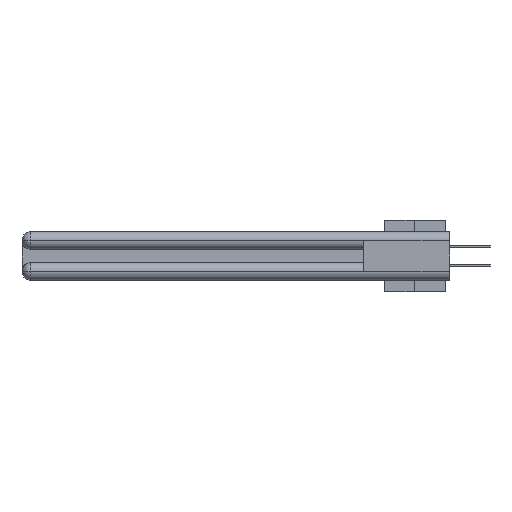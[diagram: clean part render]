
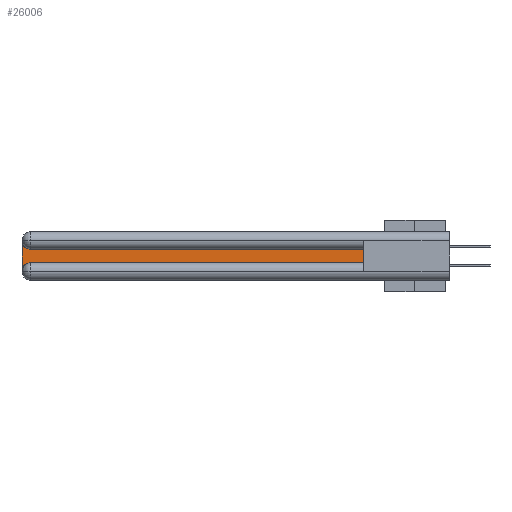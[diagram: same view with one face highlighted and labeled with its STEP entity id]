
A CAD part, left-side view. The second image highlights one B-rep face of the part: STEP entity #26006.
In plain terms, the highlighted planar face has unit normal (-1, 0, 0).
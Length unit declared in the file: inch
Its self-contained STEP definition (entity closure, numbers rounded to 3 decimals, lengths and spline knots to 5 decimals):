
#710 = PLANE ( 'NONE',  #14852 ) ;
#845 = DIRECTION ( 'NONE',  ( 1., 0., 0. ) ) ;
#1013 = EDGE_CURVE ( 'NONE', #38386, #38978, #7059, .T. ) ;
#2311 = DIRECTION ( 'NONE',  ( 1., 0., 0. ) ) ;
#3162 = ORIENTED_EDGE ( 'NONE', *, *, #1013, .T. ) ;
#3433 = VECTOR ( 'NONE', #27689, 39.37008 ) ;
#3435 = AXIS2_PLACEMENT_3D ( 'NONE', #39611, #2311, #8505 ) ;
#5744 = ORIENTED_EDGE ( 'NONE', *, *, #23359, .T. ) ;
#7059 = CIRCLE ( 'NONE', #3435, 0.06 ) ;
#7142 = CARTESIAN_POINT ( 'NONE',  ( 0.075, 3., -0.0625 ) ) ;
#8338 = DIRECTION ( 'NONE',  ( 0., 0., -1. ) ) ;
#8505 = DIRECTION ( 'NONE',  ( 0., 0., -1. ) ) ;
#8598 = CARTESIAN_POINT ( 'NONE',  ( 0.075, 0.6, -0.2175 ) ) ;
#9705 = VERTEX_POINT ( 'NONE', #8598 ) ;
#10027 = CARTESIAN_POINT ( 'NONE',  ( 0.075, 3., -0.1225 ) ) ;
#11762 = VERTEX_POINT ( 'NONE', #15130 ) ;
#12354 = EDGE_CURVE ( 'NONE', #9705, #26918, #33529, .T. ) ;
#12891 = DIRECTION ( 'NONE',  ( 0., -1., 0. ) ) ;
#14852 = AXIS2_PLACEMENT_3D ( 'NONE', #10027, #845, #31821 ) ;
#15130 = CARTESIAN_POINT ( 'NONE',  ( 0.075, 2.94, -0.2175 ) ) ;
#15148 = ORIENTED_EDGE ( 'NONE', *, *, #16966, .T. ) ;
#15164 = EDGE_CURVE ( 'NONE', #33441, #11762, #19171, .T. ) ;
#16138 = EDGE_LOOP ( 'NONE', ( #22279, #3162, #15148, #19310, #5744, #24178 ) ) ;
#16966 = EDGE_CURVE ( 'NONE', #38978, #33441, #19098, .T. ) ;
#17903 = AXIS2_PLACEMENT_3D ( 'NONE', #29203, #27306, #8338 ) ;
#19098 = LINE ( 'NONE', #36975, #3433 ) ;
#19171 = CIRCLE ( 'NONE', #17903, 0.06 ) ;
#19310 = ORIENTED_EDGE ( 'NONE', *, *, #15164, .T. ) ;
#20104 = CARTESIAN_POINT ( 'NONE',  ( 0.075, 3., -0.2775 ) ) ;
#20936 = LINE ( 'NONE', #26439, #37060 ) ;
#22279 = ORIENTED_EDGE ( 'NONE', *, *, #35531, .T. ) ;
#23154 = CARTESIAN_POINT ( 'NONE',  ( 0.075, 2.94, -0.1225 ) ) ;
#23359 = EDGE_CURVE ( 'NONE', #11762, #9705, #28509, .T. ) ;
#24178 = ORIENTED_EDGE ( 'NONE', *, *, #12354, .T. ) ;
#24619 = VECTOR ( 'NONE', #12891, 39.37008 ) ;
#25233 = CARTESIAN_POINT ( 'NONE',  ( 0.075, 0.6, -0.1225 ) ) ;
#26006 = ADVANCED_FACE ( 'NONE', ( #36746 ), #710, .F. ) ;
#26439 = CARTESIAN_POINT ( 'NONE',  ( 0.075, 0.6, -0.1225 ) ) ;
#26918 = VERTEX_POINT ( 'NONE', #25233 ) ;
#27306 = DIRECTION ( 'NONE',  ( 1., 0., 0. ) ) ;
#27516 = CARTESIAN_POINT ( 'NONE',  ( 0.075, 0.6, -0.2175 ) ) ;
#27689 = DIRECTION ( 'NONE',  ( 0., 0., -1. ) ) ;
#28509 = LINE ( 'NONE', #38287, #24619 ) ;
#29203 = CARTESIAN_POINT ( 'NONE',  ( 0.075, 2.94, -0.2775 ) ) ;
#30622 = DIRECTION ( 'NONE',  ( 0., 0., 1. ) ) ;
#31821 = DIRECTION ( 'NONE',  ( 0., 0., -1. ) ) ;
#33441 = VERTEX_POINT ( 'NONE', #20104 ) ;
#33529 = LINE ( 'NONE', #27516, #34500 ) ;
#34500 = VECTOR ( 'NONE', #30622, 39.37008 ) ;
#35531 = EDGE_CURVE ( 'NONE', #26918, #38386, #20936, .T. ) ;
#36746 = FACE_OUTER_BOUND ( 'NONE', #16138, .T. ) ;
#36975 = CARTESIAN_POINT ( 'NONE',  ( 0.075, 3., -0.2175 ) ) ;
#37060 = VECTOR ( 'NONE', #38725, 39.37008 ) ;
#38287 = CARTESIAN_POINT ( 'NONE',  ( 0.075, 0.6, -0.2175 ) ) ;
#38386 = VERTEX_POINT ( 'NONE', #23154 ) ;
#38725 = DIRECTION ( 'NONE',  ( 0., 1., 0. ) ) ;
#38978 = VERTEX_POINT ( 'NONE', #7142 ) ;
#39611 = CARTESIAN_POINT ( 'NONE',  ( 0.075, 2.94, -0.0625 ) ) ;
